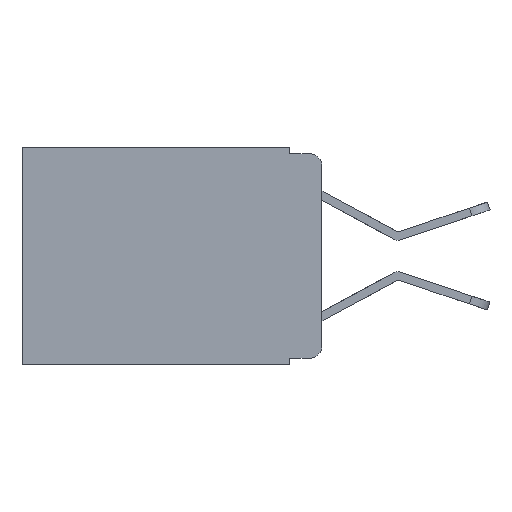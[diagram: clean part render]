
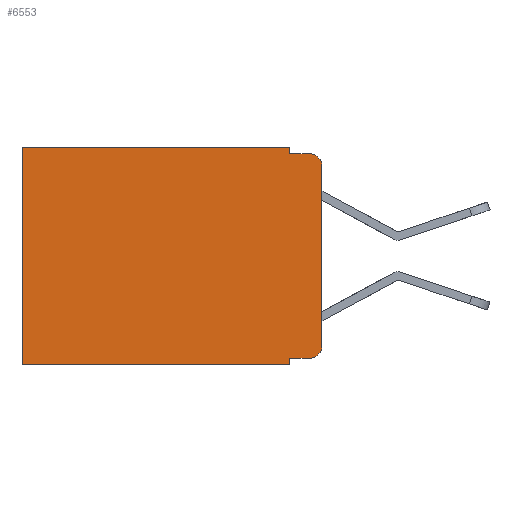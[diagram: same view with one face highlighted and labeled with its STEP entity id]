
A CAD part, left-side view. The second image highlights one B-rep face of the part: STEP entity #6553.
In plain terms, the highlighted planar face has unit normal (-1, 0, 0).
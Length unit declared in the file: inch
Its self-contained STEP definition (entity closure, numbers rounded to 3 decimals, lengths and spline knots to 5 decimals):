
#52 = ORIENTED_EDGE ( 'NONE', *, *, #3582, .F. ) ;
#179 = CARTESIAN_POINT ( 'NONE',  ( 0.298, 0.051, -0.343 ) ) ;
#453 = DIRECTION ( 'NONE',  ( 0., -1., 0. ) ) ;
#741 = CARTESIAN_POINT ( 'NONE',  ( 0.298, 0., -0.343 ) ) ;
#762 = CARTESIAN_POINT ( 'NONE',  ( 0.298, 0., 0. ) ) ;
#859 = FACE_OUTER_BOUND ( 'NONE', #3116, .T. ) ;
#881 = ORIENTED_EDGE ( 'NONE', *, *, #9361, .T. ) ;
#964 = ORIENTED_EDGE ( 'NONE', *, *, #4030, .F. ) ;
#1017 = VERTEX_POINT ( 'NONE', #5546 ) ;
#1103 = VECTOR ( 'NONE', #3524, 39.37008 ) ;
#1757 = CARTESIAN_POINT ( 'NONE',  ( 0.298, 0.051, -0.01 ) ) ;
#1894 = DIRECTION ( 'NONE',  ( 0., 0., -1. ) ) ;
#2101 = VERTEX_POINT ( 'NONE', #3799 ) ;
#2181 = ORIENTED_EDGE ( 'NONE', *, *, #2570, .T. ) ;
#2392 = VERTEX_POINT ( 'NONE', #11711 ) ;
#2515 = LINE ( 'NONE', #8936, #7612 ) ;
#2554 = CIRCLE ( 'NONE', #12576, 0.02 ) ;
#2570 = EDGE_CURVE ( 'NONE', #2392, #3860, #6389, .T. ) ;
#2590 = ORIENTED_EDGE ( 'NONE', *, *, #7424, .T. ) ;
#2744 = DIRECTION ( 'NONE',  ( 0., 0., -1. ) ) ;
#2768 = ORIENTED_EDGE ( 'NONE', *, *, #5416, .F. ) ;
#2917 = CARTESIAN_POINT ( 'NONE',  ( 0.298, 0.051, -0.01 ) ) ;
#3116 = EDGE_LOOP ( 'NONE', ( #964, #881, #2768, #4020, #2181, #2590, #52, #4526, #7058, #5469 ) ) ;
#3524 = DIRECTION ( 'NONE',  ( 0., 1., 0. ) ) ;
#3571 = CARTESIAN_POINT ( 'NONE',  ( 0.298, 0.051, -0.333 ) ) ;
#3582 = EDGE_CURVE ( 'NONE', #12396, #1017, #4215, .T. ) ;
#3621 = VECTOR ( 'NONE', #8967, 39.37008 ) ;
#3799 = CARTESIAN_POINT ( 'NONE',  ( 0.298, 0., -0.313 ) ) ;
#3860 = VERTEX_POINT ( 'NONE', #10655 ) ;
#3971 = DIRECTION ( 'NONE',  ( 0., 0., -1. ) ) ;
#4020 = ORIENTED_EDGE ( 'NONE', *, *, #6122, .F. ) ;
#4030 = EDGE_CURVE ( 'NONE', #10426, #2101, #11866, .T. ) ;
#4185 = DIRECTION ( 'NONE',  ( -1., 0., 0. ) ) ;
#4215 = LINE ( 'NONE', #741, #1103 ) ;
#4526 = ORIENTED_EDGE ( 'NONE', *, *, #6790, .F. ) ;
#4802 = CARTESIAN_POINT ( 'NONE',  ( 0.298, 0., 0. ) ) ;
#4961 = CARTESIAN_POINT ( 'NONE',  ( 0.298, 0.02, -0.313 ) ) ;
#5341 = VERTEX_POINT ( 'NONE', #1757 ) ;
#5416 = EDGE_CURVE ( 'NONE', #5341, #10297, #5654, .T. ) ;
#5433 = CARTESIAN_POINT ( 'NONE',  ( 0.298, 0., -0.03 ) ) ;
#5469 = ORIENTED_EDGE ( 'NONE', *, *, #8744, .T. ) ;
#5546 = CARTESIAN_POINT ( 'NONE',  ( 0.298, 0.473, -0.343 ) ) ;
#5602 = VERTEX_POINT ( 'NONE', #9075 ) ;
#5654 = LINE ( 'NONE', #2917, #10152 ) ;
#5857 = CARTESIAN_POINT ( 'NONE',  ( 0.298, 0.051, 0. ) ) ;
#6022 = DIRECTION ( 'NONE',  ( 0., 0., -1. ) ) ;
#6103 = DIRECTION ( 'NONE',  ( 0., 0., -1. ) ) ;
#6122 = EDGE_CURVE ( 'NONE', #2392, #5341, #9865, .T. ) ;
#6389 = LINE ( 'NONE', #9180, #3621 ) ;
#6553 = ADVANCED_FACE ( 'NONE', ( #859 ), #7156, .F. ) ;
#6638 = DIRECTION ( 'NONE',  ( 1., 0., 0. ) ) ;
#6790 = EDGE_CURVE ( 'NONE', #5602, #12396, #9705, .T. ) ;
#6908 = AXIS2_PLACEMENT_3D ( 'NONE', #4961, #11656, #6022 ) ;
#7058 = ORIENTED_EDGE ( 'NONE', *, *, #9952, .T. ) ;
#7143 = VERTEX_POINT ( 'NONE', #8548 ) ;
#7156 = PLANE ( 'NONE',  #7947 ) ;
#7236 = VECTOR ( 'NONE', #6103, 39.37008 ) ;
#7392 = CARTESIAN_POINT ( 'NONE',  ( 0.298, 0.051, 0. ) ) ;
#7424 = EDGE_CURVE ( 'NONE', #3860, #1017, #2515, .T. ) ;
#7612 = VECTOR ( 'NONE', #1894, 39.37008 ) ;
#7947 = AXIS2_PLACEMENT_3D ( 'NONE', #762, #6638, #2744 ) ;
#8139 = CARTESIAN_POINT ( 'NONE',  ( 0.298, 0.02, -0.01 ) ) ;
#8548 = CARTESIAN_POINT ( 'NONE',  ( 0.298, 0.02, -0.333 ) ) ;
#8744 = EDGE_CURVE ( 'NONE', #7143, #2101, #11720, .T. ) ;
#8936 = CARTESIAN_POINT ( 'NONE',  ( 0.298, 0.473, 0. ) ) ;
#8967 = DIRECTION ( 'NONE',  ( 0., 1., 0. ) ) ;
#9075 = CARTESIAN_POINT ( 'NONE',  ( 0.298, 0.051, -0.333 ) ) ;
#9129 = VECTOR ( 'NONE', #453, 39.37008 ) ;
#9180 = CARTESIAN_POINT ( 'NONE',  ( 0.298, 0., 0. ) ) ;
#9361 = EDGE_CURVE ( 'NONE', #10426, #10297, #2554, .T. ) ;
#9631 = DIRECTION ( 'NONE',  ( 0., -1., 0. ) ) ;
#9705 = LINE ( 'NONE', #7392, #11817 ) ;
#9865 = LINE ( 'NONE', #5857, #11701 ) ;
#9952 = EDGE_CURVE ( 'NONE', #5602, #7143, #11535, .T. ) ;
#10061 = CARTESIAN_POINT ( 'NONE',  ( 0.298, 0.02, -0.03 ) ) ;
#10152 = VECTOR ( 'NONE', #9631, 39.37008 ) ;
#10297 = VERTEX_POINT ( 'NONE', #8139 ) ;
#10426 = VERTEX_POINT ( 'NONE', #5433 ) ;
#10655 = CARTESIAN_POINT ( 'NONE',  ( 0.298, 0.473, 0. ) ) ;
#10937 = DIRECTION ( 'NONE',  ( 0., 0., -1. ) ) ;
#11535 = LINE ( 'NONE', #3571, #9129 ) ;
#11656 = DIRECTION ( 'NONE',  ( -1., 0., 0. ) ) ;
#11701 = VECTOR ( 'NONE', #11712, 39.37008 ) ;
#11711 = CARTESIAN_POINT ( 'NONE',  ( 0.298, 0.051, 0. ) ) ;
#11712 = DIRECTION ( 'NONE',  ( 0., 0., -1. ) ) ;
#11720 = CIRCLE ( 'NONE', #6908, 0.02 ) ;
#11817 = VECTOR ( 'NONE', #3971, 39.37008 ) ;
#11866 = LINE ( 'NONE', #4802, #7236 ) ;
#12396 = VERTEX_POINT ( 'NONE', #179 ) ;
#12576 = AXIS2_PLACEMENT_3D ( 'NONE', #10061, #4185, #10937 ) ;
